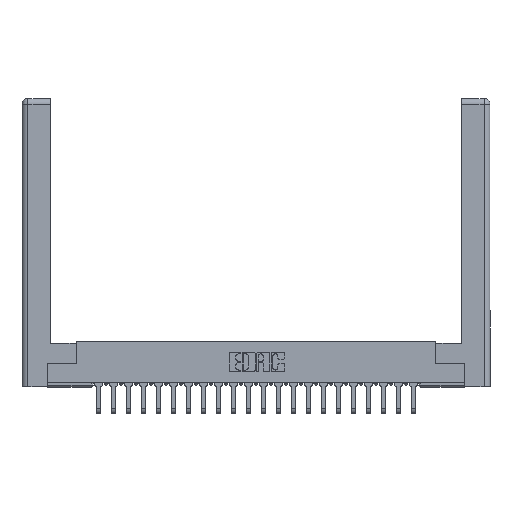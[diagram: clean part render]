
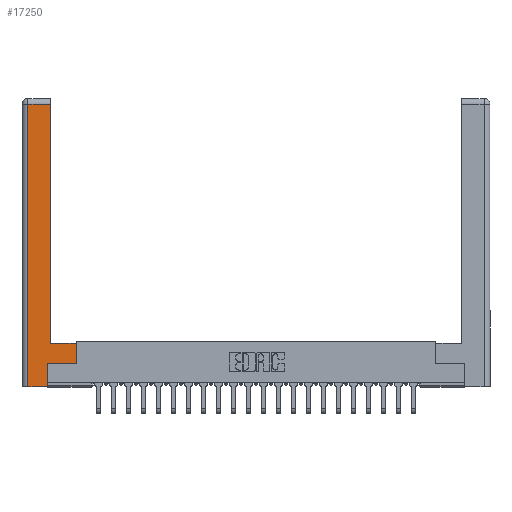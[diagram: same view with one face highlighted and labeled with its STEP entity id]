
A CAD part, top view. The second image highlights one B-rep face of the part: STEP entity #17250.
In plain terms, the highlighted planar face has unit normal (0, 0, 1).
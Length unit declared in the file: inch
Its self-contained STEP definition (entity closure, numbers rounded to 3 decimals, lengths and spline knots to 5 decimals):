
#698 = CARTESIAN_POINT ( 'NONE',  ( 0.565, 0.45, 0. ) ) ;
#842 = EDGE_CURVE ( 'NONE', #14631, #14463, #22631, .T. ) ;
#876 = VECTOR ( 'NONE', #12590, 39.37008 ) ;
#1136 = VECTOR ( 'NONE', #24855, 39.37008 ) ;
#1925 = EDGE_CURVE ( 'NONE', #7194, #11218, #12928, .T. ) ;
#2003 = EDGE_CURVE ( 'NONE', #10879, #7194, #11997, .T. ) ;
#4128 = CARTESIAN_POINT ( 'NONE',  ( 0.0615, 0., 0. ) ) ;
#4713 = CARTESIAN_POINT ( 'NONE',  ( 0., 0., 0. ) ) ;
#4810 = VECTOR ( 'NONE', #7624, 39.37008 ) ;
#4975 = VECTOR ( 'NONE', #15716, 39.37008 ) ;
#5064 = VERTEX_POINT ( 'NONE', #14364 ) ;
#5977 = EDGE_CURVE ( 'NONE', #8562, #10879, #14431, .T. ) ;
#6053 = ORIENTED_EDGE ( 'NONE', *, *, #842, .T. ) ;
#6121 = CARTESIAN_POINT ( 'NONE',  ( 0.265, 0., 0. ) ) ;
#6260 = LINE ( 'NONE', #698, #26112 ) ;
#6692 = LINE ( 'NONE', #6947, #23967 ) ;
#6763 = EDGE_CURVE ( 'NONE', #14463, #18487, #6260, .T. ) ;
#6947 = CARTESIAN_POINT ( 'NONE',  ( 0.265, 0.245, 0. ) ) ;
#7101 = EDGE_LOOP ( 'NONE', ( #15556, #25555, #17831, #13301, #25816, #6053, #8643, #9322 ) ) ;
#7194 = VERTEX_POINT ( 'NONE', #4128 ) ;
#7449 = FACE_OUTER_BOUND ( 'NONE', #7101, .T. ) ;
#7624 = DIRECTION ( 'NONE',  ( 0., 1., 0. ) ) ;
#7706 = AXIS2_PLACEMENT_3D ( 'NONE', #4713, #12793, #16897 ) ;
#7737 = CARTESIAN_POINT ( 'NONE',  ( 0.0615, 2.94, 0. ) ) ;
#8562 = VERTEX_POINT ( 'NONE', #18243 ) ;
#8643 = ORIENTED_EDGE ( 'NONE', *, *, #6763, .T. ) ;
#9052 = DIRECTION ( 'NONE',  ( 1., 0., 0. ) ) ;
#9322 = ORIENTED_EDGE ( 'NONE', *, *, #23615, .T. ) ;
#9867 = LINE ( 'NONE', #11609, #4810 ) ;
#10690 = LINE ( 'NONE', #18632, #1136 ) ;
#10879 = VERTEX_POINT ( 'NONE', #7737 ) ;
#11218 = VERTEX_POINT ( 'NONE', #6121 ) ;
#11609 = CARTESIAN_POINT ( 'NONE',  ( 0.295, 3., 0. ) ) ;
#11997 = LINE ( 'NONE', #15585, #4975 ) ;
#12590 = DIRECTION ( 'NONE',  ( 1., 0., 0. ) ) ;
#12793 = DIRECTION ( 'NONE',  ( 0., 0., -1. ) ) ;
#12928 = LINE ( 'NONE', #25093, #15369 ) ;
#13301 = ORIENTED_EDGE ( 'NONE', *, *, #1925, .T. ) ;
#13812 = VECTOR ( 'NONE', #22987, 39.37008 ) ;
#14364 = CARTESIAN_POINT ( 'NONE',  ( 0.295, 0.45, 0. ) ) ;
#14431 = LINE ( 'NONE', #22486, #13812 ) ;
#14463 = VERTEX_POINT ( 'NONE', #16624 ) ;
#14631 = VERTEX_POINT ( 'NONE', #25605 ) ;
#14641 = DIRECTION ( 'NONE',  ( 0., 1., 0. ) ) ;
#15369 = VECTOR ( 'NONE', #9052, 39.37008 ) ;
#15556 = ORIENTED_EDGE ( 'NONE', *, *, #20034, .T. ) ;
#15585 = CARTESIAN_POINT ( 'NONE',  ( 0.0615, 0., 0. ) ) ;
#15716 = DIRECTION ( 'NONE',  ( 0., -1., 0. ) ) ;
#16624 = CARTESIAN_POINT ( 'NONE',  ( 0.565, 0.245, 0. ) ) ;
#16897 = DIRECTION ( 'NONE',  ( -1., 0., 0. ) ) ;
#17250 = ADVANCED_FACE ( 'NONE', ( #7449 ), #22821, .F. ) ;
#17831 = ORIENTED_EDGE ( 'NONE', *, *, #2003, .T. ) ;
#18243 = CARTESIAN_POINT ( 'NONE',  ( 0.295, 2.94, 0. ) ) ;
#18487 = VERTEX_POINT ( 'NONE', #24697 ) ;
#18543 = CARTESIAN_POINT ( 'NONE',  ( 0.565, 0.245, 0. ) ) ;
#18632 = CARTESIAN_POINT ( 'NONE',  ( 0.295, 0.45, 0. ) ) ;
#20034 = EDGE_CURVE ( 'NONE', #5064, #8562, #9867, .T. ) ;
#22486 = CARTESIAN_POINT ( 'NONE',  ( 0.0615, 2.94, 0. ) ) ;
#22631 = LINE ( 'NONE', #18543, #876 ) ;
#22821 = PLANE ( 'NONE',  #7706 ) ;
#22899 = DIRECTION ( 'NONE',  ( 0., 1., 0. ) ) ;
#22987 = DIRECTION ( 'NONE',  ( -1., 0., 0. ) ) ;
#23615 = EDGE_CURVE ( 'NONE', #18487, #5064, #10690, .T. ) ;
#23967 = VECTOR ( 'NONE', #14641, 39.37008 ) ;
#24697 = CARTESIAN_POINT ( 'NONE',  ( 0.565, 0.45, 0. ) ) ;
#24855 = DIRECTION ( 'NONE',  ( -1., 0., 0. ) ) ;
#25093 = CARTESIAN_POINT ( 'NONE',  ( 0.265, 0., 0. ) ) ;
#25173 = EDGE_CURVE ( 'NONE', #11218, #14631, #6692, .T. ) ;
#25555 = ORIENTED_EDGE ( 'NONE', *, *, #5977, .T. ) ;
#25605 = CARTESIAN_POINT ( 'NONE',  ( 0.265, 0.245, 0. ) ) ;
#25816 = ORIENTED_EDGE ( 'NONE', *, *, #25173, .T. ) ;
#26112 = VECTOR ( 'NONE', #22899, 39.37008 ) ;
